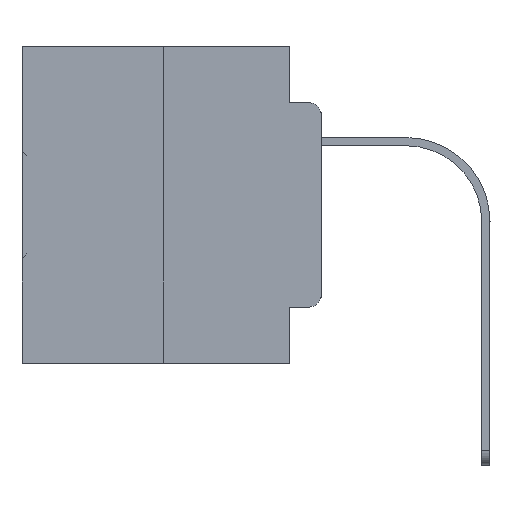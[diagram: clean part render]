
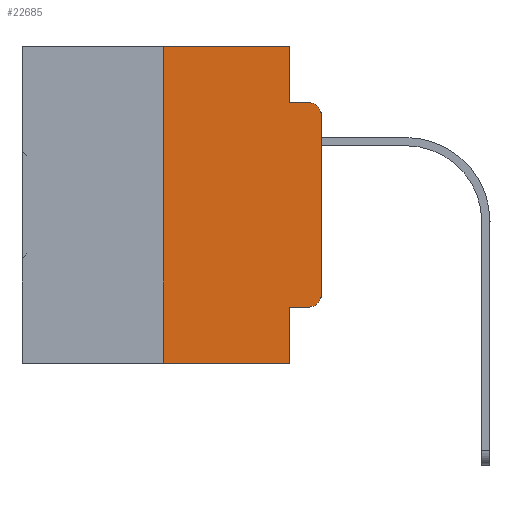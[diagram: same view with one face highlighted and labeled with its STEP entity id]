
A CAD part, left-side view. The second image highlights one B-rep face of the part: STEP entity #22685.
In plain terms, the highlighted planar face has unit normal (-1, 0, 0).
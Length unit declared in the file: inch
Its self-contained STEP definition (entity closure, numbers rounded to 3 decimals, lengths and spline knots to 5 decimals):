
#265 = VECTOR ( 'NONE', #25788, 39.37008 ) ;
#360 = CARTESIAN_POINT ( 'NONE',  ( 0., 0.473, 0. ) ) ;
#681 = VECTOR ( 'NONE', #16521, 39.37008 ) ;
#1024 = DIRECTION ( 'NONE',  ( 0., 0., -1. ) ) ;
#1217 = ORIENTED_EDGE ( 'NONE', *, *, #9552, .T. ) ;
#1240 = LINE ( 'NONE', #4256, #30852 ) ;
#1759 = CARTESIAN_POINT ( 'NONE',  ( 0., 0.051, -0.0885 ) ) ;
#2604 = ORIENTED_EDGE ( 'NONE', *, *, #18296, .T. ) ;
#3002 = CARTESIAN_POINT ( 'NONE',  ( 0., 0.051, -0.0885 ) ) ;
#3143 = EDGE_CURVE ( 'NONE', #13813, #4186, #12503, .T. ) ;
#3162 = DIRECTION ( 'NONE',  ( 0., -1., 0. ) ) ;
#3322 = VERTEX_POINT ( 'NONE', #10961 ) ;
#3416 = EDGE_CURVE ( 'NONE', #19898, #3322, #1240, .T. ) ;
#3695 = FACE_OUTER_BOUND ( 'NONE', #11334, .T. ) ;
#3720 = ORIENTED_EDGE ( 'NONE', *, *, #29751, .F. ) ;
#3902 = VECTOR ( 'NONE', #14113, 39.37008 ) ;
#4027 = CARTESIAN_POINT ( 'NONE',  ( 0., 0.051, 0. ) ) ;
#4186 = VERTEX_POINT ( 'NONE', #10882 ) ;
#4256 = CARTESIAN_POINT ( 'NONE',  ( 0., 0.25, 0. ) ) ;
#5187 = CIRCLE ( 'NONE', #23977, 0.02 ) ;
#5207 = ORIENTED_EDGE ( 'NONE', *, *, #3416, .F. ) ;
#6040 = PLANE ( 'NONE',  #28923 ) ;
#6189 = CARTESIAN_POINT ( 'NONE',  ( 0., 0.02, -0.1085 ) ) ;
#6257 = CARTESIAN_POINT ( 'NONE',  ( 0., 0.051, 0. ) ) ;
#6760 = EDGE_CURVE ( 'NONE', #4186, #20908, #5187, .T. ) ;
#7112 = DIRECTION ( 'NONE',  ( 0., -1., 0. ) ) ;
#7838 = VERTEX_POINT ( 'NONE', #16539 ) ;
#8402 = CARTESIAN_POINT ( 'NONE',  ( 0., 0., -0.3915 ) ) ;
#9034 = VERTEX_POINT ( 'NONE', #31761 ) ;
#9552 = EDGE_CURVE ( 'NONE', #24015, #7838, #22557, .T. ) ;
#9589 = VECTOR ( 'NONE', #29895, 39.37008 ) ;
#9727 = EDGE_CURVE ( 'NONE', #20908, #24015, #20451, .T. ) ;
#10882 = CARTESIAN_POINT ( 'NONE',  ( 0., 0.02, -0.4115 ) ) ;
#10961 = CARTESIAN_POINT ( 'NONE',  ( 0., 0.25, 0. ) ) ;
#11334 = EDGE_LOOP ( 'NONE', ( #23497, #1217, #22131, #33135, #3720, #5207, #2604, #14043, #28255, #12370 ) ) ;
#11740 = EDGE_CURVE ( 'NONE', #13403, #7838, #24931, .T. ) ;
#12370 = ORIENTED_EDGE ( 'NONE', *, *, #6760, .T. ) ;
#12487 = CARTESIAN_POINT ( 'NONE',  ( 0., 0.051, -0.4115 ) ) ;
#12503 = LINE ( 'NONE', #20394, #265 ) ;
#12746 = CARTESIAN_POINT ( 'NONE',  ( 0., 0.25, -0.5 ) ) ;
#12774 = CARTESIAN_POINT ( 'NONE',  ( 0., 0.02, -0.3915 ) ) ;
#12951 = CARTESIAN_POINT ( 'NONE',  ( 0., 0., -0.1085 ) ) ;
#13401 = DIRECTION ( 'NONE',  ( 0., 0., 1. ) ) ;
#13403 = VERTEX_POINT ( 'NONE', #3002 ) ;
#13788 = CARTESIAN_POINT ( 'NONE',  ( 0., 0.473, 0. ) ) ;
#13813 = VERTEX_POINT ( 'NONE', #12487 ) ;
#13994 = DIRECTION ( 'NONE',  ( 0., 0., 1. ) ) ;
#14043 = ORIENTED_EDGE ( 'NONE', *, *, #28220, .F. ) ;
#14113 = DIRECTION ( 'NONE',  ( 0., -1., 0. ) ) ;
#15626 = DIRECTION ( 'NONE',  ( 0., 0., -1. ) ) ;
#16411 = CARTESIAN_POINT ( 'NONE',  ( 0., 0.473, -0.5 ) ) ;
#16521 = DIRECTION ( 'NONE',  ( 0., 0., -1. ) ) ;
#16539 = CARTESIAN_POINT ( 'NONE',  ( 0., 0.02, -0.0885 ) ) ;
#18296 = EDGE_CURVE ( 'NONE', #19898, #21585, #18418, .T. ) ;
#18418 = LINE ( 'NONE', #16411, #25465 ) ;
#19214 = VECTOR ( 'NONE', #7112, 39.37008 ) ;
#19465 = LINE ( 'NONE', #13788, #3902 ) ;
#19871 = VECTOR ( 'NONE', #13401, 39.37008 ) ;
#19898 = VERTEX_POINT ( 'NONE', #12746 ) ;
#20394 = CARTESIAN_POINT ( 'NONE',  ( 0., 0.051, -0.4115 ) ) ;
#20451 = LINE ( 'NONE', #26002, #19871 ) ;
#20908 = VERTEX_POINT ( 'NONE', #8402 ) ;
#21585 = VERTEX_POINT ( 'NONE', #24646 ) ;
#22131 = ORIENTED_EDGE ( 'NONE', *, *, #11740, .F. ) ;
#22557 = CIRCLE ( 'NONE', #23663, 0.02 ) ;
#22685 = ADVANCED_FACE ( 'NONE', ( #3695 ), #6040, .F. ) ;
#23018 = DIRECTION ( 'NONE',  ( -1., 0., 0. ) ) ;
#23361 = DIRECTION ( 'NONE',  ( 1., 0., 0. ) ) ;
#23497 = ORIENTED_EDGE ( 'NONE', *, *, #9727, .T. ) ;
#23663 = AXIS2_PLACEMENT_3D ( 'NONE', #6189, #26535, #1024 ) ;
#23977 = AXIS2_PLACEMENT_3D ( 'NONE', #12774, #23018, #15626 ) ;
#24015 = VERTEX_POINT ( 'NONE', #12951 ) ;
#24166 = EDGE_CURVE ( 'NONE', #9034, #13403, #29396, .T. ) ;
#24412 = LINE ( 'NONE', #6257, #681 ) ;
#24646 = CARTESIAN_POINT ( 'NONE',  ( 0., 0.051, -0.5 ) ) ;
#24931 = LINE ( 'NONE', #1759, #19214 ) ;
#25465 = VECTOR ( 'NONE', #3162, 39.37008 ) ;
#25788 = DIRECTION ( 'NONE',  ( 0., -1., 0. ) ) ;
#26002 = CARTESIAN_POINT ( 'NONE',  ( 0., 0., 0. ) ) ;
#26535 = DIRECTION ( 'NONE',  ( -1., 0., 0. ) ) ;
#28220 = EDGE_CURVE ( 'NONE', #13813, #21585, #24412, .T. ) ;
#28255 = ORIENTED_EDGE ( 'NONE', *, *, #3143, .T. ) ;
#28578 = DIRECTION ( 'NONE',  ( 0., 0., -1. ) ) ;
#28923 = AXIS2_PLACEMENT_3D ( 'NONE', #360, #23361, #28578 ) ;
#29396 = LINE ( 'NONE', #4027, #9589 ) ;
#29751 = EDGE_CURVE ( 'NONE', #3322, #9034, #19465, .T. ) ;
#29895 = DIRECTION ( 'NONE',  ( 0., 0., -1. ) ) ;
#30852 = VECTOR ( 'NONE', #13994, 39.37008 ) ;
#31761 = CARTESIAN_POINT ( 'NONE',  ( 0., 0.051, 0. ) ) ;
#33135 = ORIENTED_EDGE ( 'NONE', *, *, #24166, .F. ) ;
